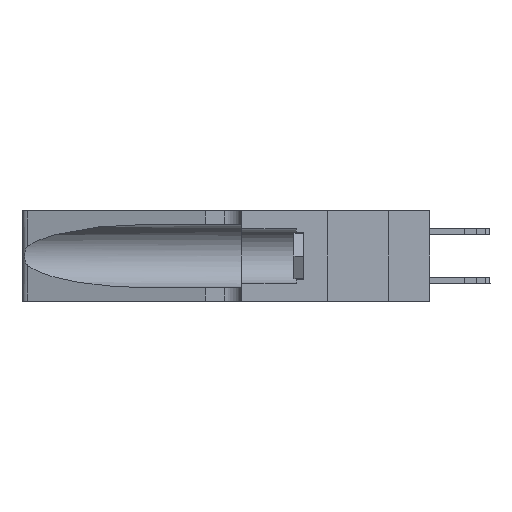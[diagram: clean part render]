
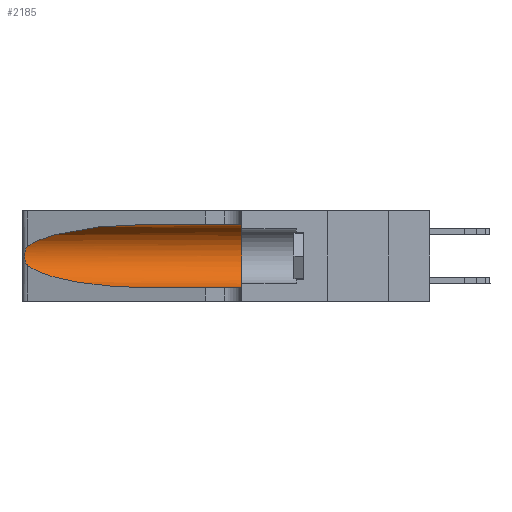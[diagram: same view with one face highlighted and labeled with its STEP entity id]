
A CAD part, left-side view. The second image highlights one B-rep face of the part: STEP entity #2185.
In plain terms, the highlighted cylindrical face has radius 3.308 mm (diameter 6.617 mm), a partial arc.
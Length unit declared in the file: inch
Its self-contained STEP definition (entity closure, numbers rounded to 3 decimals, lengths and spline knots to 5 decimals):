
#261 = AXIS2_PLACEMENT_3D ( 'NONE', #29069, #10775, #10461 ) ;
#298 = CARTESIAN_POINT ( 'NONE',  ( 0.25639, 1.23184, 0.21858 ) ) ;
#1170 = CARTESIAN_POINT ( 'NONE',  ( 0.1305, 1.61858, 0.185 ) ) ;
#1264 = ORIENTED_EDGE ( 'NONE', *, *, #8441, .F. ) ;
#1368 = DIRECTION ( 'NONE',  ( 0., -1., 0. ) ) ;
#2142 = CARTESIAN_POINT ( 'NONE',  ( 0.25487, 1.22718, 0.22369 ) ) ;
#2185 = ADVANCED_FACE ( 'NONE', ( #3480 ), #20489, .F. ) ;
#2713 = ORIENTED_EDGE ( 'NONE', *, *, #29506, .T. ) ;
#2957 =( BOUNDED_CURVE ( )  B_SPLINE_CURVE ( 3, ( #12437, #26686, #12831, #28700 ),
 .UNSPECIFIED., .F., .T. ) 
 B_SPLINE_CURVE_WITH_KNOTS ( ( 4, 4 ),
 ( 1.5708, 2.84003 ),
 .UNSPECIFIED. ) 
 CURVE ( )  GEOMETRIC_REPRESENTATION_ITEM ( )  RATIONAL_B_SPLINE_CURVE ( ( 1., 0.87, 0.87, 1. ) ) 
 REPRESENTATION_ITEM ( '' )  );
#3395 = DIRECTION ( 'NONE',  ( 0., -1., 0. ) ) ;
#3480 = FACE_OUTER_BOUND ( 'NONE', #19077, .T. ) ;
#5395 = VERTEX_POINT ( 'NONE', #16909 ) ;
#5792 = VERTEX_POINT ( 'NONE', #23658 ) ;
#5949 = CARTESIAN_POINT ( 'NONE',  ( 0.26018, 1.23835, 0.19895 ) ) ;
#6053 = CARTESIAN_POINT ( 'NONE',  ( 0.25856, 1.23593, 0.16098 ) ) ;
#7325 = CARTESIAN_POINT ( 'NONE',  ( 0.1305, 1.61858, 0.05475 ) ) ;
#7414 = CARTESIAN_POINT ( 'NONE',  ( 0.25555, 1.22994, 0.2215 ) ) ;
#7910 = LINE ( 'NONE', #17062, #18043 ) ;
#8314 = EDGE_CURVE ( 'NONE', #14776, #5792, #10341, .T. ) ;
#8441 = EDGE_CURVE ( 'NONE', #29121, #26740, #7910, .T. ) ;
#9304 = CARTESIAN_POINT ( 'NONE',  ( 0.18966, 0.96281, 0.05475 ) ) ;
#9932 = LINE ( 'NONE', #7325, #26236 ) ;
#10341 = B_SPLINE_CURVE_WITH_KNOTS ( 'NONE', 3,
 ( #18564, #7414, #298, #24888, #17478, #5949, #29438, #24472, #20099, #6053, #19995, #26819, #29126, #13775 ),
 .UNSPECIFIED., .F., .F.,
 ( 4, 2, 2, 2, 2, 2, 4 ),
 ( 0., 0.00027, 0.00053, 0.00107, 0.0016, 0.00187, 0.00214 ),
 .UNSPECIFIED. ) ;
#10461 = DIRECTION ( 'NONE',  ( 0., 0., 1. ) ) ;
#10603 =( BOUNDED_CURVE ( )  B_SPLINE_CURVE ( 3, ( #23176, #23270, #9304, #27921 ),
 .UNSPECIFIED., .F., .F. ) 
 B_SPLINE_CURVE_WITH_KNOTS ( ( 4, 4 ),
 ( 3.44316, 4.71239 ),
 .UNSPECIFIED. ) 
 CURVE ( )  GEOMETRIC_REPRESENTATION_ITEM ( )  RATIONAL_B_SPLINE_CURVE ( ( 1., 0.87, 0.87, 1. ) ) 
 REPRESENTATION_ITEM ( '' )  );
#10775 = DIRECTION ( 'NONE',  ( 0., 1., 0. ) ) ;
#11270 = CIRCLE ( 'NONE', #261, 0.13025 ) ;
#11368 = ORIENTED_EDGE ( 'NONE', *, *, #15540, .T. ) ;
#12221 = DIRECTION ( 'NONE',  ( 0., -1., 0. ) ) ;
#12437 = CARTESIAN_POINT ( 'NONE',  ( 0.1305, 0.72297, 0.31525 ) ) ;
#12831 = CARTESIAN_POINT ( 'NONE',  ( 0.2373, 1.15595, 0.28018 ) ) ;
#13775 = CARTESIAN_POINT ( 'NONE',  ( 0.25487, 1.22718, 0.14631 ) ) ;
#14336 = ORIENTED_EDGE ( 'NONE', *, *, #25722, .F. ) ;
#14776 = VERTEX_POINT ( 'NONE', #2142 ) ;
#15540 = EDGE_CURVE ( 'NONE', #5792, #5395, #10603, .T. ) ;
#16909 = CARTESIAN_POINT ( 'NONE',  ( 0.1305, 0.72297, 0.05475 ) ) ;
#17062 = CARTESIAN_POINT ( 'NONE',  ( 0.1305, 1.61858, 0.31525 ) ) ;
#17478 = CARTESIAN_POINT ( 'NONE',  ( 0.25854, 1.2359, 0.20912 ) ) ;
#18043 = VECTOR ( 'NONE', #3395, 39.37008 ) ;
#18564 = CARTESIAN_POINT ( 'NONE',  ( 0.25487, 1.22718, 0.22369 ) ) ;
#19077 = EDGE_LOOP ( 'NONE', ( #23689, #26154, #11368, #2713, #14336, #1264 ) ) ;
#19774 = DIRECTION ( 'NONE',  ( 0., 0., -1. ) ) ;
#19995 = CARTESIAN_POINT ( 'NONE',  ( 0.25789, 1.23486, 0.15765 ) ) ;
#20071 = CARTESIAN_POINT ( 'NONE',  ( 0.1305, 0.35, 0.31525 ) ) ;
#20099 = CARTESIAN_POINT ( 'NONE',  ( 0.26017, 1.23833, 0.17102 ) ) ;
#20294 = EDGE_CURVE ( 'NONE', #29121, #14776, #2957, .T. ) ;
#20489 = CYLINDRICAL_SURFACE ( 'NONE', #26271, 0.13025 ) ;
#23176 = CARTESIAN_POINT ( 'NONE',  ( 0.25487, 1.22718, 0.14631 ) ) ;
#23270 = CARTESIAN_POINT ( 'NONE',  ( 0.2373, 1.15595, 0.08982 ) ) ;
#23658 = CARTESIAN_POINT ( 'NONE',  ( 0.25487, 1.22718, 0.14631 ) ) ;
#23689 = ORIENTED_EDGE ( 'NONE', *, *, #20294, .T. ) ;
#24472 = CARTESIAN_POINT ( 'NONE',  ( 0.26075, 1.23896, 0.178 ) ) ;
#24888 = CARTESIAN_POINT ( 'NONE',  ( 0.25787, 1.23484, 0.2124 ) ) ;
#25722 = EDGE_CURVE ( 'NONE', #26740, #28402, #11270, .T. ) ;
#26154 = ORIENTED_EDGE ( 'NONE', *, *, #8314, .T. ) ;
#26236 = VECTOR ( 'NONE', #12221, 39.37008 ) ;
#26271 = AXIS2_PLACEMENT_3D ( 'NONE', #1170, #1368, #19774 ) ;
#26686 = CARTESIAN_POINT ( 'NONE',  ( 0.18966, 0.96281, 0.31525 ) ) ;
#26740 = VERTEX_POINT ( 'NONE', #20071 ) ;
#26819 = CARTESIAN_POINT ( 'NONE',  ( 0.25639, 1.23186, 0.15144 ) ) ;
#27921 = CARTESIAN_POINT ( 'NONE',  ( 0.1305, 0.72297, 0.05475 ) ) ;
#28402 = VERTEX_POINT ( 'NONE', #28808 ) ;
#28700 = CARTESIAN_POINT ( 'NONE',  ( 0.25487, 1.22718, 0.22369 ) ) ;
#28808 = CARTESIAN_POINT ( 'NONE',  ( 0.1305, 0.35, 0.05475 ) ) ;
#29069 = CARTESIAN_POINT ( 'NONE',  ( 0.1305, 0.35, 0.185 ) ) ;
#29121 = VERTEX_POINT ( 'NONE', #29123 ) ;
#29123 = CARTESIAN_POINT ( 'NONE',  ( 0.1305, 0.72297, 0.31525 ) ) ;
#29126 = CARTESIAN_POINT ( 'NONE',  ( 0.25555, 1.22993, 0.14849 ) ) ;
#29438 = CARTESIAN_POINT ( 'NONE',  ( 0.26075, 1.23896, 0.19203 ) ) ;
#29506 = EDGE_CURVE ( 'NONE', #5395, #28402, #9932, .T. ) ;
